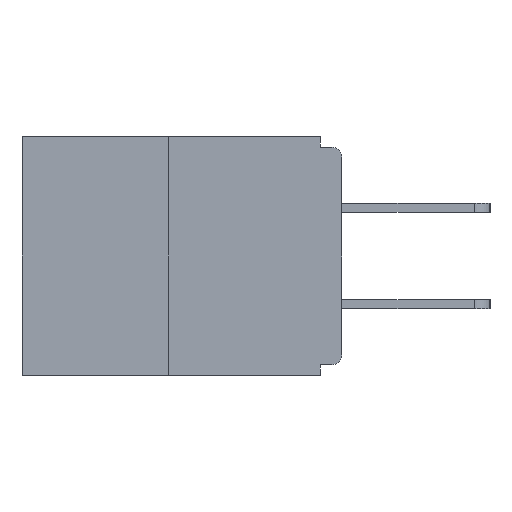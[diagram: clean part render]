
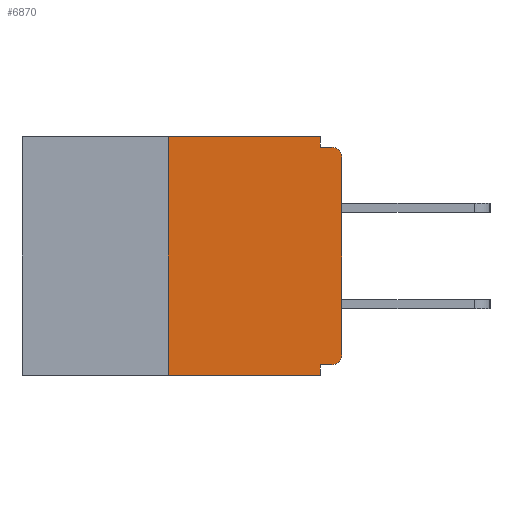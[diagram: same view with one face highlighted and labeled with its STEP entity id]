
A CAD part, left-side view. The second image highlights one B-rep face of the part: STEP entity #6870.
In plain terms, the highlighted planar face has unit normal (-1, 0, 0).
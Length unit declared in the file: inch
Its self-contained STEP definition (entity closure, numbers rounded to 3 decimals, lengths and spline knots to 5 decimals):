
#193 = CARTESIAN_POINT ( 'NONE',  ( 0., 0.015, -0.03 ) ) ;
#241 = EDGE_CURVE ( 'NONE', #3388, #2464, #11523, .T. ) ;
#421 = DIRECTION ( 'NONE',  ( 0., 0., -1. ) ) ;
#516 = DIRECTION ( 'NONE',  ( 1., 0., 0. ) ) ;
#567 = CARTESIAN_POINT ( 'NONE',  ( 0., 0.25, 0. ) ) ;
#718 = VECTOR ( 'NONE', #7538, 39.37008 ) ;
#1565 = CARTESIAN_POINT ( 'NONE',  ( 0., 0., -0.328 ) ) ;
#1639 = CARTESIAN_POINT ( 'NONE',  ( 0., 0.015, -0.313 ) ) ;
#1745 = DIRECTION ( 'NONE',  ( 0., -1., 0. ) ) ;
#1751 = EDGE_CURVE ( 'NONE', #10340, #9081, #4433, .T. ) ;
#1982 = VECTOR ( 'NONE', #5972, 39.37008 ) ;
#2229 = EDGE_CURVE ( 'NONE', #10834, #9081, #4600, .T. ) ;
#2367 = CARTESIAN_POINT ( 'NONE',  ( 0., 0., -0.015 ) ) ;
#2464 = VERTEX_POINT ( 'NONE', #10490 ) ;
#2619 = CARTESIAN_POINT ( 'NONE',  ( 0., 0.031, 0. ) ) ;
#2750 = DIRECTION ( 'NONE',  ( 0., 1., 0. ) ) ;
#2813 = CARTESIAN_POINT ( 'NONE',  ( 0., 0.015, -0.328 ) ) ;
#2828 = DIRECTION ( 'NONE',  ( 0., 0., -1. ) ) ;
#3178 = ORIENTED_EDGE ( 'NONE', *, *, #5425, .F. ) ;
#3388 = VERTEX_POINT ( 'NONE', #8494 ) ;
#3864 = VERTEX_POINT ( 'NONE', #2619 ) ;
#3870 = DIRECTION ( 'NONE',  ( -1., 0., 0. ) ) ;
#4402 = ORIENTED_EDGE ( 'NONE', *, *, #9567, .T. ) ;
#4433 = CIRCLE ( 'NONE', #4516, 0.015 ) ;
#4495 = AXIS2_PLACEMENT_3D ( 'NONE', #1639, #3870, #2828 ) ;
#4516 = AXIS2_PLACEMENT_3D ( 'NONE', #193, #13108, #4592 ) ;
#4526 = VERTEX_POINT ( 'NONE', #11540 ) ;
#4541 = ORIENTED_EDGE ( 'NONE', *, *, #241, .T. ) ;
#4575 = VECTOR ( 'NONE', #1745, 39.37008 ) ;
#4592 = DIRECTION ( 'NONE',  ( 0., 0., -1. ) ) ;
#4600 = LINE ( 'NONE', #2367, #5113 ) ;
#4706 = CARTESIAN_POINT ( 'NONE',  ( 0., 0.031, -0.015 ) ) ;
#4726 = ORIENTED_EDGE ( 'NONE', *, *, #5157, .F. ) ;
#4749 = CARTESIAN_POINT ( 'NONE',  ( 0., 0.031, -0.343 ) ) ;
#4849 = CARTESIAN_POINT ( 'NONE',  ( 0., 0.25, 0. ) ) ;
#5113 = VECTOR ( 'NONE', #8866, 39.37008 ) ;
#5157 = EDGE_CURVE ( 'NONE', #3864, #10834, #5393, .T. ) ;
#5246 = CARTESIAN_POINT ( 'NONE',  ( 0., 0.031, 0. ) ) ;
#5332 = ORIENTED_EDGE ( 'NONE', *, *, #1751, .T. ) ;
#5342 = FACE_OUTER_BOUND ( 'NONE', #7915, .T. ) ;
#5393 = LINE ( 'NONE', #5246, #7100 ) ;
#5425 = EDGE_CURVE ( 'NONE', #3388, #6166, #7381, .T. ) ;
#5474 = EDGE_CURVE ( 'NONE', #11192, #2464, #5560, .T. ) ;
#5560 = LINE ( 'NONE', #4749, #13572 ) ;
#5972 = DIRECTION ( 'NONE',  ( 0., -1., 0. ) ) ;
#6166 = VERTEX_POINT ( 'NONE', #567 ) ;
#6870 = ADVANCED_FACE ( 'NONE', ( #5342 ), #7919, .F. ) ;
#6963 = CARTESIAN_POINT ( 'NONE',  ( 0., 0., -0.03 ) ) ;
#6985 = DIRECTION ( 'NONE',  ( 0., 0., 1. ) ) ;
#7100 = VECTOR ( 'NONE', #8469, 39.37008 ) ;
#7101 = ORIENTED_EDGE ( 'NONE', *, *, #13045, .F. ) ;
#7355 = VERTEX_POINT ( 'NONE', #2813 ) ;
#7381 = LINE ( 'NONE', #4849, #11231 ) ;
#7538 = DIRECTION ( 'NONE',  ( 0., 0., 1. ) ) ;
#7915 = EDGE_LOOP ( 'NONE', ( #10577, #3178, #4541, #11124, #7101, #4402, #9171, #5332, #8523, #4726 ) ) ;
#7919 = PLANE ( 'NONE',  #12629 ) ;
#8111 = CIRCLE ( 'NONE', #4495, 0.015 ) ;
#8316 = CARTESIAN_POINT ( 'NONE',  ( 0., 0.46, 0. ) ) ;
#8442 = LINE ( 'NONE', #1565, #9775 ) ;
#8469 = DIRECTION ( 'NONE',  ( 0., 0., -1. ) ) ;
#8494 = CARTESIAN_POINT ( 'NONE',  ( 0., 0.25, -0.343 ) ) ;
#8523 = ORIENTED_EDGE ( 'NONE', *, *, #2229, .F. ) ;
#8866 = DIRECTION ( 'NONE',  ( 0., -1., 0. ) ) ;
#9081 = VERTEX_POINT ( 'NONE', #12997 ) ;
#9110 = DIRECTION ( 'NONE',  ( 0., 0., -1. ) ) ;
#9171 = ORIENTED_EDGE ( 'NONE', *, *, #10058, .T. ) ;
#9391 = EDGE_CURVE ( 'NONE', #6166, #3864, #11604, .T. ) ;
#9567 = EDGE_CURVE ( 'NONE', #7355, #4526, #8111, .T. ) ;
#9668 = CARTESIAN_POINT ( 'NONE',  ( 0., 0., 0. ) ) ;
#9775 = VECTOR ( 'NONE', #2750, 39.37008 ) ;
#10058 = EDGE_CURVE ( 'NONE', #4526, #10340, #11287, .T. ) ;
#10340 = VERTEX_POINT ( 'NONE', #6963 ) ;
#10490 = CARTESIAN_POINT ( 'NONE',  ( 0., 0.031, -0.343 ) ) ;
#10577 = ORIENTED_EDGE ( 'NONE', *, *, #9391, .F. ) ;
#10834 = VERTEX_POINT ( 'NONE', #4706 ) ;
#11124 = ORIENTED_EDGE ( 'NONE', *, *, #5474, .F. ) ;
#11192 = VERTEX_POINT ( 'NONE', #11984 ) ;
#11231 = VECTOR ( 'NONE', #6985, 39.37008 ) ;
#11287 = LINE ( 'NONE', #9668, #718 ) ;
#11315 = CARTESIAN_POINT ( 'NONE',  ( 0., 0.46, 0. ) ) ;
#11523 = LINE ( 'NONE', #12344, #1982 ) ;
#11540 = CARTESIAN_POINT ( 'NONE',  ( 0., 0., -0.313 ) ) ;
#11604 = LINE ( 'NONE', #8316, #4575 ) ;
#11984 = CARTESIAN_POINT ( 'NONE',  ( 0., 0.031, -0.328 ) ) ;
#12344 = CARTESIAN_POINT ( 'NONE',  ( 0., 0.46, -0.343 ) ) ;
#12629 = AXIS2_PLACEMENT_3D ( 'NONE', #11315, #516, #421 ) ;
#12997 = CARTESIAN_POINT ( 'NONE',  ( 0., 0.015, -0.015 ) ) ;
#13045 = EDGE_CURVE ( 'NONE', #7355, #11192, #8442, .T. ) ;
#13108 = DIRECTION ( 'NONE',  ( -1., 0., 0. ) ) ;
#13572 = VECTOR ( 'NONE', #9110, 39.37008 ) ;
